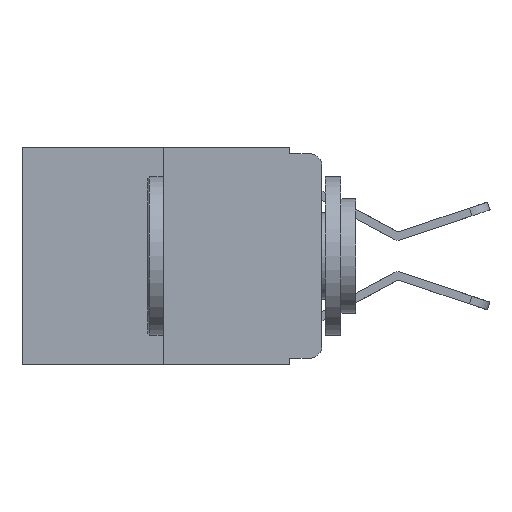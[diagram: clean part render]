
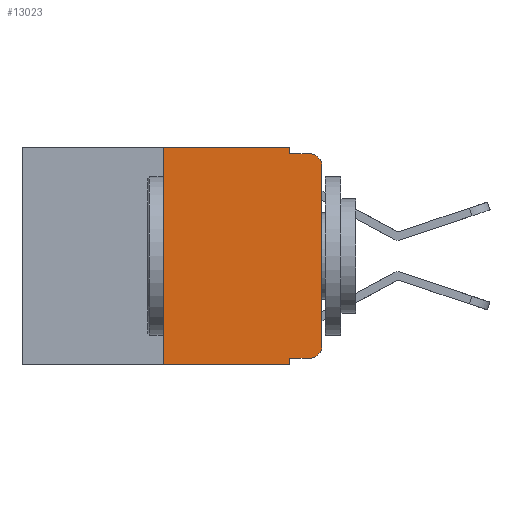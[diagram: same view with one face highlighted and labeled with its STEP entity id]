
A CAD part, left-side view. The second image highlights one B-rep face of the part: STEP entity #13023.
In plain terms, the highlighted planar face has unit normal (-1, 0, 0).
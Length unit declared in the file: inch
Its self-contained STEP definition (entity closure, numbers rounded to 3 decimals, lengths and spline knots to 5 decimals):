
#783 = AXIS2_PLACEMENT_3D ( 'NONE', #16895, #6590, #9572 ) ;
#853 = PLANE ( 'NONE',  #3346 ) ;
#934 = DIRECTION ( 'NONE',  ( -1., 0., 0. ) ) ;
#1158 = VECTOR ( 'NONE', #6060, 39.37008 ) ;
#1232 = VECTOR ( 'NONE', #3669, 39.37008 ) ;
#1279 = EDGE_CURVE ( 'NONE', #10988, #2223, #13195, .T. ) ;
#1514 = CIRCLE ( 'NONE', #2129, 0.02 ) ;
#1661 = CARTESIAN_POINT ( 'NONE',  ( 0., 0.25, 0. ) ) ;
#1809 = DIRECTION ( 'NONE',  ( 0., -1., 0. ) ) ;
#2034 = CARTESIAN_POINT ( 'NONE',  ( 0., 0.051, 0. ) ) ;
#2129 = AXIS2_PLACEMENT_3D ( 'NONE', #17007, #934, #12592 ) ;
#2155 = VERTEX_POINT ( 'NONE', #2741 ) ;
#2223 = VERTEX_POINT ( 'NONE', #11518 ) ;
#2468 = ORIENTED_EDGE ( 'NONE', *, *, #17170, .T. ) ;
#2628 = VECTOR ( 'NONE', #9039, 39.37008 ) ;
#2741 = CARTESIAN_POINT ( 'NONE',  ( 0., 0.051, -0.01 ) ) ;
#2797 = ORIENTED_EDGE ( 'NONE', *, *, #17335, .T. ) ;
#2856 = EDGE_CURVE ( 'NONE', #4924, #5755, #10706, .T. ) ;
#3121 = VECTOR ( 'NONE', #9245, 39.37008 ) ;
#3293 = DIRECTION ( 'NONE',  ( 0., 0., -1. ) ) ;
#3346 = AXIS2_PLACEMENT_3D ( 'NONE', #16588, #16487, #3293 ) ;
#3377 = CARTESIAN_POINT ( 'NONE',  ( 0., 0.051, -0.333 ) ) ;
#3595 = VERTEX_POINT ( 'NONE', #6574 ) ;
#3669 = DIRECTION ( 'NONE',  ( 0., 0., -1. ) ) ;
#4924 = VERTEX_POINT ( 'NONE', #9297 ) ;
#5089 = CARTESIAN_POINT ( 'NONE',  ( 0., 0.473, -0.343 ) ) ;
#5247 = VECTOR ( 'NONE', #7115, 39.37008 ) ;
#5497 = EDGE_CURVE ( 'NONE', #4924, #3595, #18730, .T. ) ;
#5722 = CIRCLE ( 'NONE', #783, 0.02 ) ;
#5743 = CARTESIAN_POINT ( 'NONE',  ( 0., 0.25, 0. ) ) ;
#5755 = VERTEX_POINT ( 'NONE', #15525 ) ;
#5816 = ORIENTED_EDGE ( 'NONE', *, *, #9026, .F. ) ;
#6060 = DIRECTION ( 'NONE',  ( 0., -1., 0. ) ) ;
#6516 = LINE ( 'NONE', #5089, #15351 ) ;
#6574 = CARTESIAN_POINT ( 'NONE',  ( 0., 0.051, -0.343 ) ) ;
#6590 = DIRECTION ( 'NONE',  ( -1., 0., 0. ) ) ;
#6815 = ORIENTED_EDGE ( 'NONE', *, *, #5497, .F. ) ;
#6885 = LINE ( 'NONE', #5743, #7135 ) ;
#7115 = DIRECTION ( 'NONE',  ( 0., 0., 1. ) ) ;
#7135 = VECTOR ( 'NONE', #9685, 39.37008 ) ;
#7159 = CARTESIAN_POINT ( 'NONE',  ( 0., 0.051, 0. ) ) ;
#7502 = CARTESIAN_POINT ( 'NONE',  ( 0., 0., 0. ) ) ;
#7582 = CARTESIAN_POINT ( 'NONE',  ( 0., 0.473, 0. ) ) ;
#8293 = VECTOR ( 'NONE', #12862, 39.37008 ) ;
#8770 = VERTEX_POINT ( 'NONE', #15056 ) ;
#9026 = EDGE_CURVE ( 'NONE', #2155, #14031, #9225, .T. ) ;
#9039 = DIRECTION ( 'NONE',  ( 0., -1., 0. ) ) ;
#9225 = LINE ( 'NONE', #13388, #2628 ) ;
#9245 = DIRECTION ( 'NONE',  ( 0., -1., 0. ) ) ;
#9297 = CARTESIAN_POINT ( 'NONE',  ( 0., 0.051, -0.333 ) ) ;
#9429 = EDGE_CURVE ( 'NONE', #8770, #14031, #5722, .T. ) ;
#9497 = CARTESIAN_POINT ( 'NONE',  ( 0., 0., -0.313 ) ) ;
#9572 = DIRECTION ( 'NONE',  ( 0., 0., -1. ) ) ;
#9685 = DIRECTION ( 'NONE',  ( 0., 0., 1. ) ) ;
#10410 = CARTESIAN_POINT ( 'NONE',  ( 0., 0.02, -0.01 ) ) ;
#10706 = LINE ( 'NONE', #3377, #3121 ) ;
#10721 = FACE_OUTER_BOUND ( 'NONE', #18705, .T. ) ;
#10988 = VERTEX_POINT ( 'NONE', #1661 ) ;
#11055 = ORIENTED_EDGE ( 'NONE', *, *, #9429, .T. ) ;
#11518 = CARTESIAN_POINT ( 'NONE',  ( 0., 0.051, 0. ) ) ;
#12322 = EDGE_CURVE ( 'NONE', #12741, #10988, #6885, .T. ) ;
#12592 = DIRECTION ( 'NONE',  ( 0., 0., -1. ) ) ;
#12741 = VERTEX_POINT ( 'NONE', #18432 ) ;
#12834 = ORIENTED_EDGE ( 'NONE', *, *, #1279, .F. ) ;
#12862 = DIRECTION ( 'NONE',  ( 0., 0., -1. ) ) ;
#13023 = ADVANCED_FACE ( 'NONE', ( #10721 ), #853, .F. ) ;
#13195 = LINE ( 'NONE', #7582, #1158 ) ;
#13388 = CARTESIAN_POINT ( 'NONE',  ( 0., 0.051, -0.01 ) ) ;
#13560 = VERTEX_POINT ( 'NONE', #9497 ) ;
#14031 = VERTEX_POINT ( 'NONE', #10410 ) ;
#14913 = ORIENTED_EDGE ( 'NONE', *, *, #17807, .F. ) ;
#15056 = CARTESIAN_POINT ( 'NONE',  ( 0., 0., -0.03 ) ) ;
#15351 = VECTOR ( 'NONE', #1809, 39.37008 ) ;
#15525 = CARTESIAN_POINT ( 'NONE',  ( 0., 0.02, -0.333 ) ) ;
#15989 = LINE ( 'NONE', #7502, #5247 ) ;
#16487 = DIRECTION ( 'NONE',  ( 1., 0., 0. ) ) ;
#16588 = CARTESIAN_POINT ( 'NONE',  ( 0., 0.473, 0. ) ) ;
#16895 = CARTESIAN_POINT ( 'NONE',  ( 0., 0.02, -0.03 ) ) ;
#16952 = ORIENTED_EDGE ( 'NONE', *, *, #18419, .T. ) ;
#17007 = CARTESIAN_POINT ( 'NONE',  ( 0., 0.02, -0.313 ) ) ;
#17141 = ORIENTED_EDGE ( 'NONE', *, *, #12322, .F. ) ;
#17170 = EDGE_CURVE ( 'NONE', #12741, #3595, #6516, .T. ) ;
#17335 = EDGE_CURVE ( 'NONE', #5755, #13560, #1514, .T. ) ;
#17807 = EDGE_CURVE ( 'NONE', #2223, #2155, #18311, .T. ) ;
#17962 = ORIENTED_EDGE ( 'NONE', *, *, #2856, .T. ) ;
#18311 = LINE ( 'NONE', #2034, #1232 ) ;
#18419 = EDGE_CURVE ( 'NONE', #13560, #8770, #15989, .T. ) ;
#18432 = CARTESIAN_POINT ( 'NONE',  ( 0., 0.25, -0.343 ) ) ;
#18705 = EDGE_LOOP ( 'NONE', ( #16952, #11055, #5816, #14913, #12834, #17141, #2468, #6815, #17962, #2797 ) ) ;
#18730 = LINE ( 'NONE', #7159, #8293 ) ;
